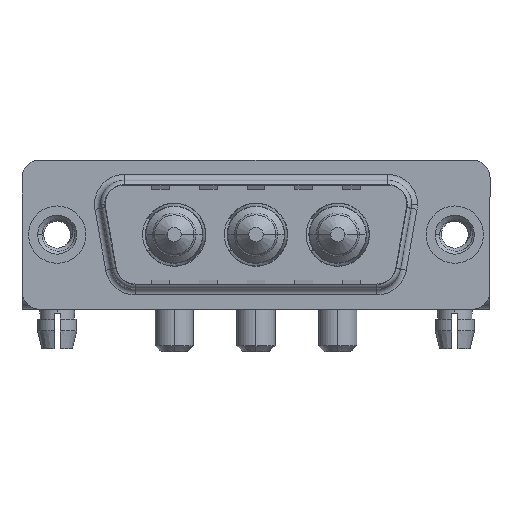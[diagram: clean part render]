
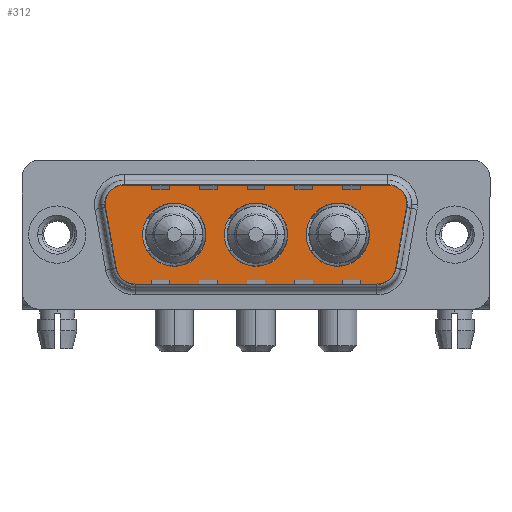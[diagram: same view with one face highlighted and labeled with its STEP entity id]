
A CAD part, top view. The second image highlights one B-rep face of the part: STEP entity #312.
In plain terms, the highlighted planar face has unit normal (0, 0, 1).
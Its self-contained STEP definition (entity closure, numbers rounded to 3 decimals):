
#75 = PLANE ( 'NONE',  #7506 ) ;
#249 = DIRECTION ( 'NONE',  ( 0., 0., 1. ) ) ;
#297 = DIRECTION ( 'NONE',  ( 0., 0., 1. ) ) ;
#312 = ADVANCED_FACE ( 'NONE', ( #5953, #9391, #7109, #11878 ), #75, .T. ) ;
#340 = DIRECTION ( 'NONE',  ( 1., 0., 0. ) ) ;
#347 = VERTEX_POINT ( 'NONE', #10572 ) ;
#467 = VECTOR ( 'NONE', #6618, 1000. ) ;
#573 = AXIS2_PLACEMENT_3D ( 'NONE', #3843, #8627, #340 ) ;
#707 = AXIS2_PLACEMENT_3D ( 'NONE', #15413, #11900, #5663 ) ;
#751 = DIRECTION ( 'NONE',  ( 0.174, 0.985, 0. ) ) ;
#898 = AXIS2_PLACEMENT_3D ( 'NONE', #7572, #1316, #8665 ) ;
#1024 = DIRECTION ( 'NONE',  ( 0., 0., 1. ) ) ;
#1047 = VERTEX_POINT ( 'NONE', #3444 ) ;
#1139 = CIRCLE ( 'NONE', #7124, 2.65 ) ;
#1173 = CARTESIAN_POINT ( 'NONE',  ( 26.866, -2.9, 0. ) ) ;
#1316 = DIRECTION ( 'NONE',  ( 0., 0., 1. ) ) ;
#1432 = CARTESIAN_POINT ( 'NONE',  ( 6.434, -4.9, 0. ) ) ;
#1659 = CIRCLE ( 'NONE', #898, 2.65 ) ;
#1773 = ORIENTED_EDGE ( 'NONE', *, *, #9489, .F. ) ;
#1847 = LINE ( 'NONE', #4340, #12913 ) ;
#1917 = CARTESIAN_POINT ( 'NONE',  ( 5.411, 4.9, 0. ) ) ;
#2085 = ORIENTED_EDGE ( 'NONE', *, *, #12989, .T. ) ;
#2253 = VERTEX_POINT ( 'NONE', #7255 ) ;
#2319 = EDGE_CURVE ( 'NONE', #11682, #7644, #11304, .T. ) ;
#2371 = CARTESIAN_POINT ( 'NONE',  ( 6.434, -4.9, 0. ) ) ;
#2473 = DIRECTION ( 'NONE',  ( -1., 0., 0. ) ) ;
#2595 = DIRECTION ( 'NONE',  ( 0., 0., 1. ) ) ;
#3051 = CIRCLE ( 'NONE', #11783, 2.65 ) ;
#3277 = VERTEX_POINT ( 'NONE', #4703 ) ;
#3289 = EDGE_CURVE ( 'NONE', #6992, #1047, #3051, .T. ) ;
#3311 = EDGE_CURVE ( 'NONE', #8196, #2253, #12135, .T. ) ;
#3380 = AXIS2_PLACEMENT_3D ( 'NONE', #4696, #249, #3520 ) ;
#3412 = ORIENTED_EDGE ( 'NONE', *, *, #6578, .T. ) ;
#3444 = CARTESIAN_POINT ( 'NONE',  ( 7.15, 0., 0. ) ) ;
#3469 = EDGE_CURVE ( 'NONE', #7406, #5270, #14796, .T. ) ;
#3520 = DIRECTION ( 'NONE',  ( 1., 0., 0. ) ) ;
#3661 = CARTESIAN_POINT ( 'NONE',  ( 28.836, -3.247, 0. ) ) ;
#3774 = ORIENTED_EDGE ( 'NONE', *, *, #10866, .T. ) ;
#3843 = CARTESIAN_POINT ( 'NONE',  ( 23.5, 0., 0. ) ) ;
#3861 = CARTESIAN_POINT ( 'NONE',  ( 16.65, 0., 0. ) ) ;
#3931 = ORIENTED_EDGE ( 'NONE', *, *, #12304, .T. ) ;
#4033 = LINE ( 'NONE', #6472, #467 ) ;
#4173 = AXIS2_PLACEMENT_3D ( 'NONE', #13457, #6591, #12522 ) ;
#4340 = CARTESIAN_POINT ( 'NONE',  ( 29.859, 2.553, 0. ) ) ;
#4361 = DIRECTION ( 'NONE',  ( -1., 0., 0. ) ) ;
#4589 = DIRECTION ( 'NONE',  ( 0., 0., 1. ) ) ;
#4696 = CARTESIAN_POINT ( 'NONE',  ( 9.8, 0., 0. ) ) ;
#4703 = CARTESIAN_POINT ( 'NONE',  ( 4.464, -3.247, 0. ) ) ;
#4842 = DIRECTION ( 'NONE',  ( 1., 0., 0. ) ) ;
#4956 = DIRECTION ( 'NONE',  ( 1., 0., 0. ) ) ;
#5095 = LINE ( 'NONE', #12582, #13860 ) ;
#5260 = CARTESIAN_POINT ( 'NONE',  ( 27.889, 2.9, 0. ) ) ;
#5270 = VERTEX_POINT ( 'NONE', #12306 ) ;
#5663 = DIRECTION ( 'NONE',  ( -1., 0., 0. ) ) ;
#5701 = CARTESIAN_POINT ( 'NONE',  ( 5.411, 2.9, 0. ) ) ;
#5945 = EDGE_CURVE ( 'NONE', #7571, #3277, #4033, .T. ) ;
#5953 = FACE_BOUND ( 'NONE', #14086, .T. ) ;
#6013 = VERTEX_POINT ( 'NONE', #1917 ) ;
#6227 = ORIENTED_EDGE ( 'NONE', *, *, #14574, .F. ) ;
#6250 = CARTESIAN_POINT ( 'NONE',  ( 27.889, 2.9, 0. ) ) ;
#6328 = ORIENTED_EDGE ( 'NONE', *, *, #3311, .T. ) ;
#6445 = CIRCLE ( 'NONE', #4173, 2. ) ;
#6472 = CARTESIAN_POINT ( 'NONE',  ( 3.441, 2.553, 0. ) ) ;
#6578 = EDGE_CURVE ( 'NONE', #11268, #347, #1847, .T. ) ;
#6591 = DIRECTION ( 'NONE',  ( 0., 0., 1. ) ) ;
#6618 = DIRECTION ( 'NONE',  ( 0.174, -0.985, 0. ) ) ;
#6720 = DIRECTION ( 'NONE',  ( 1., 0., 0. ) ) ;
#6750 = CARTESIAN_POINT ( 'NONE',  ( 19.3, 0., 0. ) ) ;
#6992 = VERTEX_POINT ( 'NONE', #11136 ) ;
#7106 = VERTEX_POINT ( 'NONE', #6750 ) ;
#7109 = FACE_BOUND ( 'NONE', #13386, .T. ) ;
#7124 = AXIS2_PLACEMENT_3D ( 'NONE', #3861, #12151, #4956 ) ;
#7255 = CARTESIAN_POINT ( 'NONE',  ( 26.866, -4.9, 0. ) ) ;
#7406 = VERTEX_POINT ( 'NONE', #9479 ) ;
#7453 = CIRCLE ( 'NONE', #707, 2. ) ;
#7506 = AXIS2_PLACEMENT_3D ( 'NONE', #1173, #1024, #4842 ) ;
#7559 = EDGE_CURVE ( 'NONE', #7644, #6013, #5095, .T. ) ;
#7571 = VERTEX_POINT ( 'NONE', #14709 ) ;
#7572 = CARTESIAN_POINT ( 'NONE',  ( 23.5, 0., 0. ) ) ;
#7644 = VERTEX_POINT ( 'NONE', #12951 ) ;
#7723 = AXIS2_PLACEMENT_3D ( 'NONE', #5260, #12446, #8790 ) ;
#7817 = AXIS2_PLACEMENT_3D ( 'NONE', #6250, #297, #2473 ) ;
#7897 = EDGE_CURVE ( 'NONE', #5270, #7406, #1659, .T. ) ;
#7910 = ORIENTED_EDGE ( 'NONE', *, *, #2319, .T. ) ;
#8196 = VERTEX_POINT ( 'NONE', #2371 ) ;
#8336 = VERTEX_POINT ( 'NONE', #12236 ) ;
#8627 = DIRECTION ( 'NONE',  ( 0., 0., 1. ) ) ;
#8665 = DIRECTION ( 'NONE',  ( 1., 0., 0. ) ) ;
#8790 = DIRECTION ( 'NONE',  ( -1., 0., 0. ) ) ;
#8923 = ORIENTED_EDGE ( 'NONE', *, *, #11994, .T. ) ;
#9022 = EDGE_CURVE ( 'NONE', #8336, #7106, #1139, .T. ) ;
#9049 = EDGE_LOOP ( 'NONE', ( #3774, #3412, #3931, #7910, #10356, #2085, #13927, #8923, #6328 ) ) ;
#9146 = ORIENTED_EDGE ( 'NONE', *, *, #7897, .F. ) ;
#9391 = FACE_BOUND ( 'NONE', #15045, .T. ) ;
#9479 = CARTESIAN_POINT ( 'NONE',  ( 20.85, 0., 0. ) ) ;
#9489 = EDGE_CURVE ( 'NONE', #1047, #6992, #15110, .T. ) ;
#9689 = ORIENTED_EDGE ( 'NONE', *, *, #9022, .F. ) ;
#9900 = CARTESIAN_POINT ( 'NONE',  ( 16.65, 0., 0. ) ) ;
#10115 = DIRECTION ( 'NONE',  ( 1., 0., 0. ) ) ;
#10251 = CARTESIAN_POINT ( 'NONE',  ( 29.889, 2.9, 0. ) ) ;
#10356 = ORIENTED_EDGE ( 'NONE', *, *, #7559, .T. ) ;
#10485 = DIRECTION ( 'NONE',  ( 1., 0., 0. ) ) ;
#10572 = CARTESIAN_POINT ( 'NONE',  ( 29.859, 2.553, 0. ) ) ;
#10866 = EDGE_CURVE ( 'NONE', #2253, #11268, #6445, .T. ) ;
#11136 = CARTESIAN_POINT ( 'NONE',  ( 12.45, 0., 0. ) ) ;
#11232 = CIRCLE ( 'NONE', #14467, 2. ) ;
#11268 = VERTEX_POINT ( 'NONE', #3661 ) ;
#11304 = CIRCLE ( 'NONE', #7817, 2. ) ;
#11682 = VERTEX_POINT ( 'NONE', #10251 ) ;
#11715 = ORIENTED_EDGE ( 'NONE', *, *, #3469, .F. ) ;
#11783 = AXIS2_PLACEMENT_3D ( 'NONE', #13307, #2595, #15412 ) ;
#11878 = FACE_OUTER_BOUND ( 'NONE', #9049, .T. ) ;
#11900 = DIRECTION ( 'NONE',  ( 0., 0., 1. ) ) ;
#11994 = EDGE_CURVE ( 'NONE', #3277, #8196, #7453, .T. ) ;
#12135 = LINE ( 'NONE', #1432, #13775 ) ;
#12151 = DIRECTION ( 'NONE',  ( 0., 0., 1. ) ) ;
#12236 = CARTESIAN_POINT ( 'NONE',  ( 14., 0., 0. ) ) ;
#12304 = EDGE_CURVE ( 'NONE', #347, #11682, #14182, .T. ) ;
#12306 = CARTESIAN_POINT ( 'NONE',  ( 26.15, 0., 0. ) ) ;
#12446 = DIRECTION ( 'NONE',  ( 0., 0., 1. ) ) ;
#12470 = CIRCLE ( 'NONE', #14201, 2.65 ) ;
#12522 = DIRECTION ( 'NONE',  ( 1., 0., 0. ) ) ;
#12582 = CARTESIAN_POINT ( 'NONE',  ( 5.411, 4.9, 0. ) ) ;
#12913 = VECTOR ( 'NONE', #751, 1000. ) ;
#12951 = CARTESIAN_POINT ( 'NONE',  ( 27.889, 4.9, 0. ) ) ;
#12989 = EDGE_CURVE ( 'NONE', #6013, #7571, #11232, .T. ) ;
#13307 = CARTESIAN_POINT ( 'NONE',  ( 9.8, 0., 0. ) ) ;
#13386 = EDGE_LOOP ( 'NONE', ( #13950, #1773 ) ) ;
#13457 = CARTESIAN_POINT ( 'NONE',  ( 26.866, -2.9, 0. ) ) ;
#13775 = VECTOR ( 'NONE', #10115, 1000. ) ;
#13860 = VECTOR ( 'NONE', #4361, 1000. ) ;
#13927 = ORIENTED_EDGE ( 'NONE', *, *, #5945, .T. ) ;
#13950 = ORIENTED_EDGE ( 'NONE', *, *, #3289, .F. ) ;
#14086 = EDGE_LOOP ( 'NONE', ( #6227, #9689 ) ) ;
#14182 = CIRCLE ( 'NONE', #7723, 2. ) ;
#14201 = AXIS2_PLACEMENT_3D ( 'NONE', #9900, #14649, #10485 ) ;
#14467 = AXIS2_PLACEMENT_3D ( 'NONE', #5701, #4589, #6720 ) ;
#14574 = EDGE_CURVE ( 'NONE', #7106, #8336, #12470, .T. ) ;
#14649 = DIRECTION ( 'NONE',  ( 0., 0., 1. ) ) ;
#14709 = CARTESIAN_POINT ( 'NONE',  ( 3.441, 2.553, 0. ) ) ;
#14796 = CIRCLE ( 'NONE', #573, 2.65 ) ;
#15045 = EDGE_LOOP ( 'NONE', ( #9146, #11715 ) ) ;
#15110 = CIRCLE ( 'NONE', #3380, 2.65 ) ;
#15412 = DIRECTION ( 'NONE',  ( 1., 0., 0. ) ) ;
#15413 = CARTESIAN_POINT ( 'NONE',  ( 6.434, -2.9, 0. ) ) ;
